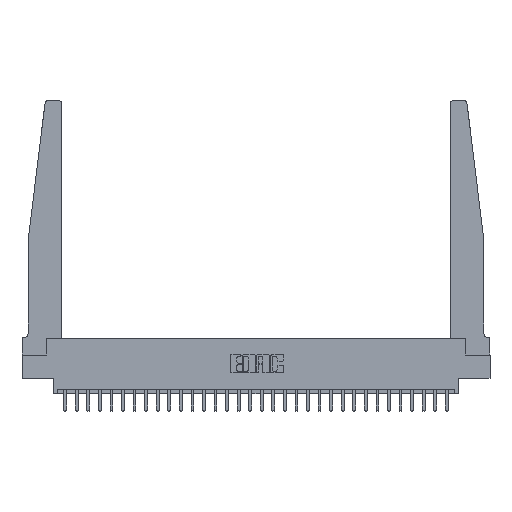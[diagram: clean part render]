
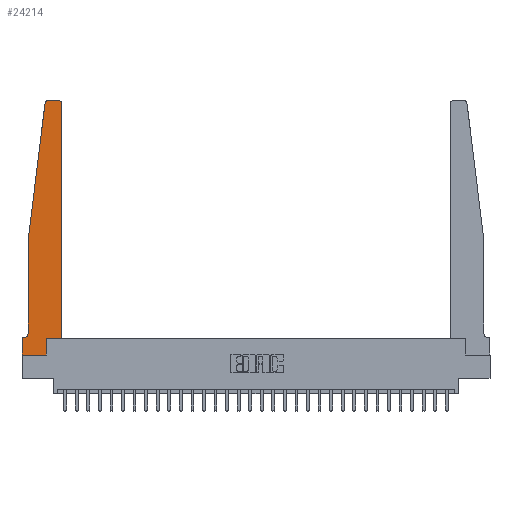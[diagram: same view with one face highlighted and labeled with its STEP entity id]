
A CAD part, top view. The second image highlights one B-rep face of the part: STEP entity #24214.
In plain terms, the highlighted planar face has unit normal (0, 0, 1).
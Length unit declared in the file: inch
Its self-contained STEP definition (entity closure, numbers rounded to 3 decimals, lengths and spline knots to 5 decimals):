
#508 = EDGE_LOOP ( 'NONE', ( #19387, #7828, #4340, #14378, #25390, #4142, #10100, #10079, #20192, #24141, #2046, #6544 ) ) ;
#772 = VECTOR ( 'NONE', #22807, 39.37008 ) ;
#1369 = DIRECTION ( 'NONE',  ( 0., 0., 1. ) ) ;
#1686 = LINE ( 'NONE', #5638, #6894 ) ;
#1770 = VERTEX_POINT ( 'NONE', #20493 ) ;
#1818 = CARTESIAN_POINT ( 'NONE',  ( 0., 0., 0.37 ) ) ;
#2046 = ORIENTED_EDGE ( 'NONE', *, *, #24094, .T. ) ;
#2397 = VECTOR ( 'NONE', #7866, 39.37008 ) ;
#3012 = CARTESIAN_POINT ( 'NONE',  ( 0., 0., 0.37 ) ) ;
#3057 = CARTESIAN_POINT ( 'NONE',  ( 0.065, 1.25, 0.37 ) ) ;
#3425 = PLANE ( 'NONE',  #8281 ) ;
#3964 = FACE_OUTER_BOUND ( 'NONE', #508, .T. ) ;
#4142 = ORIENTED_EDGE ( 'NONE', *, *, #9026, .T. ) ;
#4340 = ORIENTED_EDGE ( 'NONE', *, *, #14317, .T. ) ;
#4438 = CARTESIAN_POINT ( 'NONE',  ( 0.2605, 0., 0.37 ) ) ;
#5076 = EDGE_CURVE ( 'NONE', #14921, #20641, #8256, .T. ) ;
#5489 = CARTESIAN_POINT ( 'NONE',  ( 0.065, 0.1875, 0.37 ) ) ;
#5638 = CARTESIAN_POINT ( 'NONE',  ( 0.065, 1.25, 0.37 ) ) ;
#5732 = DIRECTION ( 'NONE',  ( -0.122, -0.992, 0. ) ) ;
#5835 = EDGE_CURVE ( 'NONE', #17122, #12345, #14018, .T. ) ;
#6281 = VERTEX_POINT ( 'NONE', #22292 ) ;
#6511 = CARTESIAN_POINT ( 'NONE',  ( 0.2605, 0.18, 0.37 ) ) ;
#6544 = ORIENTED_EDGE ( 'NONE', *, *, #8717, .T. ) ;
#6596 = CARTESIAN_POINT ( 'NONE',  ( 0.395, 2.75, 0.37 ) ) ;
#6661 = LINE ( 'NONE', #6511, #772 ) ;
#6739 = VECTOR ( 'NONE', #25036, 39.37008 ) ;
#6778 = EDGE_CURVE ( 'NONE', #14153, #15800, #20165, .T. ) ;
#6870 = LINE ( 'NONE', #3057, #13450 ) ;
#6894 = VECTOR ( 'NONE', #5732, 39.37008 ) ;
#6963 = CARTESIAN_POINT ( 'NONE',  ( 0.065, 0.2375, 0.37 ) ) ;
#7429 = LINE ( 'NONE', #14218, #6739 ) ;
#7828 = ORIENTED_EDGE ( 'NONE', *, *, #5076, .T. ) ;
#7866 = DIRECTION ( 'NONE',  ( 1., 0., 0. ) ) ;
#7961 = CARTESIAN_POINT ( 'NONE',  ( 0.27653, 2.72, 0.37 ) ) ;
#8142 = VECTOR ( 'NONE', #16222, 39.37008 ) ;
#8256 = CIRCLE ( 'NONE', #21548, 0.03 ) ;
#8281 = AXIS2_PLACEMENT_3D ( 'NONE', #23244, #1369, #16796 ) ;
#8717 = EDGE_CURVE ( 'NONE', #19946, #14591, #9805, .T. ) ;
#9026 = EDGE_CURVE ( 'NONE', #15800, #27252, #24755, .T. ) ;
#9087 = CARTESIAN_POINT ( 'NONE',  ( 0.015, 0.2375, 0.37 ) ) ;
#9282 = EDGE_CURVE ( 'NONE', #14591, #14921, #14202, .T. ) ;
#9805 = CIRCLE ( 'NONE', #13055, 0.03 ) ;
#9892 = CARTESIAN_POINT ( 'NONE',  ( 0.27653, 2.75, 0.37 ) ) ;
#10079 = ORIENTED_EDGE ( 'NONE', *, *, #5835, .T. ) ;
#10100 = ORIENTED_EDGE ( 'NONE', *, *, #18138, .T. ) ;
#10196 = DIRECTION ( 'NONE',  ( 1., 0., 0. ) ) ;
#10521 = CARTESIAN_POINT ( 'NONE',  ( 0.015, 0.1875, 0.37 ) ) ;
#11242 = CARTESIAN_POINT ( 'NONE',  ( 0.395, 2.72, 0.37 ) ) ;
#11314 = DIRECTION ( 'NONE',  ( -1., 0., 0. ) ) ;
#12345 = VERTEX_POINT ( 'NONE', #4438 ) ;
#12358 = VERTEX_POINT ( 'NONE', #13437 ) ;
#13055 = AXIS2_PLACEMENT_3D ( 'NONE', #11242, #26411, #13439 ) ;
#13262 = CARTESIAN_POINT ( 'NONE',  ( 0., 0.1875, 0.37 ) ) ;
#13437 = CARTESIAN_POINT ( 'NONE',  ( 0.425, 0.18, 0.37 ) ) ;
#13439 = DIRECTION ( 'NONE',  ( 1., 0., 0. ) ) ;
#13450 = VECTOR ( 'NONE', #18456, 39.37008 ) ;
#14018 = LINE ( 'NONE', #3012, #8142 ) ;
#14153 = VERTEX_POINT ( 'NONE', #6963 ) ;
#14202 = LINE ( 'NONE', #21781, #25071 ) ;
#14218 = CARTESIAN_POINT ( 'NONE',  ( 0.425, 0.18, 0.37 ) ) ;
#14284 = EDGE_CURVE ( 'NONE', #1770, #12358, #19245, .T. ) ;
#14297 = LINE ( 'NONE', #16995, #25164 ) ;
#14317 = EDGE_CURVE ( 'NONE', #20641, #6281, #1686, .T. ) ;
#14378 = ORIENTED_EDGE ( 'NONE', *, *, #15522, .T. ) ;
#14591 = VERTEX_POINT ( 'NONE', #6596 ) ;
#14921 = VERTEX_POINT ( 'NONE', #9892 ) ;
#15092 = CARTESIAN_POINT ( 'NONE',  ( 0.24675, 2.72367, 0.37 ) ) ;
#15522 = EDGE_CURVE ( 'NONE', #6281, #14153, #6870, .T. ) ;
#15800 = VERTEX_POINT ( 'NONE', #10521 ) ;
#16222 = DIRECTION ( 'NONE',  ( 1., 0., 0. ) ) ;
#16458 = DIRECTION ( 'NONE',  ( -1., 0., 0. ) ) ;
#16796 = DIRECTION ( 'NONE',  ( 1., 0., 0. ) ) ;
#16995 = CARTESIAN_POINT ( 'NONE',  ( 0., 0., 0.37 ) ) ;
#17122 = VERTEX_POINT ( 'NONE', #1818 ) ;
#18138 = EDGE_CURVE ( 'NONE', #27252, #17122, #14297, .T. ) ;
#18456 = DIRECTION ( 'NONE',  ( 0., -1., 0. ) ) ;
#19187 = DIRECTION ( 'NONE',  ( 0., -1., 0. ) ) ;
#19245 = LINE ( 'NONE', #20984, #2397 ) ;
#19387 = ORIENTED_EDGE ( 'NONE', *, *, #9282, .T. ) ;
#19946 = VERTEX_POINT ( 'NONE', #23739 ) ;
#20165 = CIRCLE ( 'NONE', #26471, 0.05 ) ;
#20192 = ORIENTED_EDGE ( 'NONE', *, *, #26499, .T. ) ;
#20493 = CARTESIAN_POINT ( 'NONE',  ( 0.2605, 0.18, 0.37 ) ) ;
#20641 = VERTEX_POINT ( 'NONE', #15092 ) ;
#20984 = CARTESIAN_POINT ( 'NONE',  ( 0.425, 0.18, 0.37 ) ) ;
#21548 = AXIS2_PLACEMENT_3D ( 'NONE', #7961, #23238, #10196 ) ;
#21781 = CARTESIAN_POINT ( 'NONE',  ( 0.25, 2.75, 0.37 ) ) ;
#22292 = CARTESIAN_POINT ( 'NONE',  ( 0.065, 1.25, 0.37 ) ) ;
#22807 = DIRECTION ( 'NONE',  ( 0., 1., 0. ) ) ;
#23238 = DIRECTION ( 'NONE',  ( 0., 0., 1. ) ) ;
#23244 = CARTESIAN_POINT ( 'NONE',  ( 0., 0.1875, 0.37 ) ) ;
#23739 = CARTESIAN_POINT ( 'NONE',  ( 0.425, 2.72, 0.37 ) ) ;
#23936 = DIRECTION ( 'NONE',  ( -1., 0., 0. ) ) ;
#24094 = EDGE_CURVE ( 'NONE', #12358, #19946, #7429, .T. ) ;
#24141 = ORIENTED_EDGE ( 'NONE', *, *, #14284, .T. ) ;
#24214 = ADVANCED_FACE ( 'NONE', ( #3964 ), #3425, .T. ) ;
#24330 = DIRECTION ( 'NONE',  ( 0., 0., -1. ) ) ;
#24755 = LINE ( 'NONE', #5489, #25422 ) ;
#25036 = DIRECTION ( 'NONE',  ( 0., 1., 0. ) ) ;
#25071 = VECTOR ( 'NONE', #23936, 39.37008 ) ;
#25164 = VECTOR ( 'NONE', #19187, 39.37008 ) ;
#25390 = ORIENTED_EDGE ( 'NONE', *, *, #6778, .T. ) ;
#25422 = VECTOR ( 'NONE', #16458, 39.37008 ) ;
#26411 = DIRECTION ( 'NONE',  ( 0., 0., 1. ) ) ;
#26471 = AXIS2_PLACEMENT_3D ( 'NONE', #9087, #24330, #11314 ) ;
#26499 = EDGE_CURVE ( 'NONE', #12345, #1770, #6661, .T. ) ;
#27252 = VERTEX_POINT ( 'NONE', #13262 ) ;
